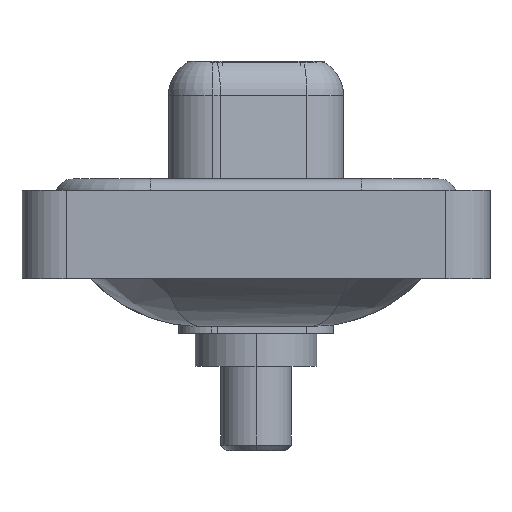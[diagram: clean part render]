
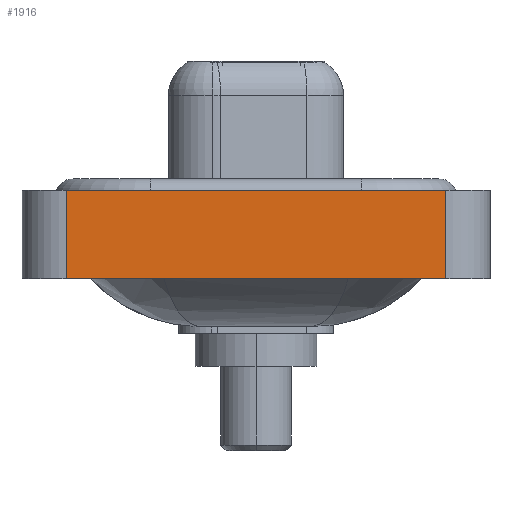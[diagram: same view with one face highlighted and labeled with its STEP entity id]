
A CAD part, left-side view. The second image highlights one B-rep face of the part: STEP entity #1916.
In plain terms, the highlighted planar face has unit normal (-1, 0, 0).
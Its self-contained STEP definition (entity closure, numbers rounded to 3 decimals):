
#122 = EDGE_CURVE ( 'NONE', #12381, #9462, #11714, .T. ) ;
#631 = DIRECTION ( 'NONE',  ( 0., 0., 1. ) ) ;
#856 = VECTOR ( 'NONE', #631, 1000. ) ;
#1154 = VECTOR ( 'NONE', #3911, 1000. ) ;
#1218 = VERTEX_POINT ( 'NONE', #5603 ) ;
#1916 = ADVANCED_FACE ( 'NONE', ( #3715 ), #7276, .T. ) ;
#2520 = CARTESIAN_POINT ( 'NONE',  ( -7.25, -8.55, -3.6 ) ) ;
#2968 = CARTESIAN_POINT ( 'NONE',  ( -7.25, 8.55, -3.6 ) ) ;
#3575 = EDGE_LOOP ( 'NONE', ( #13005, #4722, #12995, #4321 ) ) ;
#3715 = FACE_OUTER_BOUND ( 'NONE', #3575, .T. ) ;
#3911 = DIRECTION ( 'NONE',  ( 0., -1., 0. ) ) ;
#4197 = AXIS2_PLACEMENT_3D ( 'NONE', #7506, #8530, #10998 ) ;
#4321 = ORIENTED_EDGE ( 'NONE', *, *, #122, .T. ) ;
#4722 = ORIENTED_EDGE ( 'NONE', *, *, #5510, .F. ) ;
#5298 = CARTESIAN_POINT ( 'NONE',  ( -7.25, 8.55, 0.4 ) ) ;
#5510 = EDGE_CURVE ( 'NONE', #6613, #1218, #10159, .T. ) ;
#5603 = CARTESIAN_POINT ( 'NONE',  ( -7.25, -8.55, 0.4 ) ) ;
#5777 = CARTESIAN_POINT ( 'NONE',  ( -7.25, -8.55, -3.6 ) ) ;
#6613 = VERTEX_POINT ( 'NONE', #5298 ) ;
#6692 = LINE ( 'NONE', #10256, #856 ) ;
#6917 = VECTOR ( 'NONE', #12892, 1000. ) ;
#6960 = EDGE_CURVE ( 'NONE', #12381, #6613, #6692, .T. ) ;
#7276 = PLANE ( 'NONE',  #4197 ) ;
#7506 = CARTESIAN_POINT ( 'NONE',  ( -7.25, -8.55, -3.6 ) ) ;
#7630 = EDGE_CURVE ( 'NONE', #9462, #1218, #12812, .T. ) ;
#8530 = DIRECTION ( 'NONE',  ( -1., 0., 0. ) ) ;
#9462 = VERTEX_POINT ( 'NONE', #2520 ) ;
#10159 = LINE ( 'NONE', #14750, #1154 ) ;
#10256 = CARTESIAN_POINT ( 'NONE',  ( -7.25, 8.55, -3.6 ) ) ;
#10998 = DIRECTION ( 'NONE',  ( 0., 0., 1. ) ) ;
#11620 = CARTESIAN_POINT ( 'NONE',  ( -7.25, -8.55, -3.6 ) ) ;
#11714 = LINE ( 'NONE', #5777, #14152 ) ;
#12381 = VERTEX_POINT ( 'NONE', #2968 ) ;
#12812 = LINE ( 'NONE', #11620, #6917 ) ;
#12826 = DIRECTION ( 'NONE',  ( 0., -1., 0. ) ) ;
#12892 = DIRECTION ( 'NONE',  ( 0., 0., 1. ) ) ;
#12995 = ORIENTED_EDGE ( 'NONE', *, *, #6960, .F. ) ;
#13005 = ORIENTED_EDGE ( 'NONE', *, *, #7630, .T. ) ;
#14152 = VECTOR ( 'NONE', #12826, 1000. ) ;
#14750 = CARTESIAN_POINT ( 'NONE',  ( -7.25, -8.55, 0.4 ) ) ;
